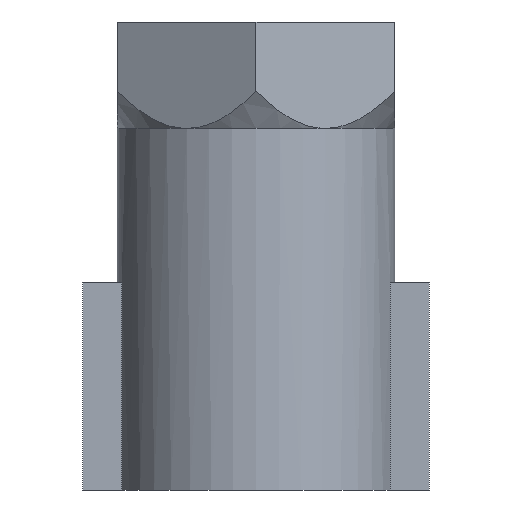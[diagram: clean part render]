
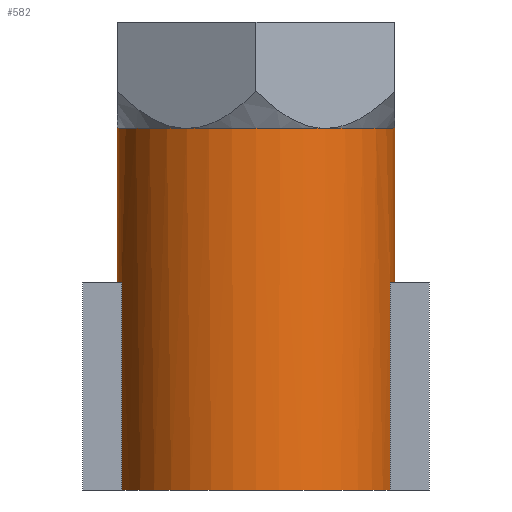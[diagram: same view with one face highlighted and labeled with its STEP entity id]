
A CAD part, front view. The second image highlights one B-rep face of the part: STEP entity #582.
In plain terms, the highlighted cylindrical face has radius 10 mm (diameter 20 mm), a partial arc.
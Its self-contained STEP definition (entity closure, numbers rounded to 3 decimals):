
#63 = VERTEX_POINT ( 'NONE', #501 ) ;
#76 = CARTESIAN_POINT ( 'NONE',  ( 10., 0., 26.075 ) ) ;
#106 = DIRECTION ( 'NONE',  ( 0., 0., -1. ) ) ;
#113 = CARTESIAN_POINT ( 'NONE',  ( 0., 0., 26.075 ) ) ;
#130 = VERTEX_POINT ( 'NONE', #152 ) ;
#152 = CARTESIAN_POINT ( 'NONE',  ( -10., 0., 15. ) ) ;
#212 = DIRECTION ( 'NONE',  ( 1., 0., 0. ) ) ;
#221 = DIRECTION ( 'NONE',  ( 0., 0., 1. ) ) ;
#224 = CARTESIAN_POINT ( 'NONE',  ( 0., 0., 15. ) ) ;
#261 = CIRCLE ( 'NONE', #816, 10. ) ;
#264 = VECTOR ( 'NONE', #981, 1000. ) ;
#270 = DIRECTION ( 'NONE',  ( 0., 0., -1. ) ) ;
#278 = CARTESIAN_POINT ( 'NONE',  ( -10., 0., 16. ) ) ;
#293 = LINE ( 'NONE', #1172, #264 ) ;
#297 = DIRECTION ( 'NONE',  ( 1., 0., 0. ) ) ;
#299 = DIRECTION ( 'NONE',  ( 0., 0., -1. ) ) ;
#300 = CARTESIAN_POINT ( 'NONE',  ( 0., 0., 26.075 ) ) ;
#306 = CARTESIAN_POINT ( 'NONE',  ( 9.682, -2.5, 16. ) ) ;
#316 = DIRECTION ( 'NONE',  ( 0., 0., 1. ) ) ;
#376 = CARTESIAN_POINT ( 'NONE',  ( -10., 0., 26.075 ) ) ;
#411 = DIRECTION ( 'NONE',  ( 1., 0., 0. ) ) ;
#418 = DIRECTION ( 'NONE',  ( 1., 0., 0. ) ) ;
#421 = DIRECTION ( 'NONE',  ( 0., 0., 1. ) ) ;
#422 = EDGE_CURVE ( 'NONE', #63, #885, #925, .T. ) ;
#438 = ORIENTED_EDGE ( 'NONE', *, *, #1187, .F. ) ;
#440 = FACE_OUTER_BOUND ( 'NONE', #640, .T. ) ;
#453 = VECTOR ( 'NONE', #1087, 1000. ) ;
#470 = ORIENTED_EDGE ( 'NONE', *, *, #744, .T. ) ;
#471 = ORIENTED_EDGE ( 'NONE', *, *, #1132, .T. ) ;
#478 = CARTESIAN_POINT ( 'NONE',  ( -9.682, -2.5, 16. ) ) ;
#494 = ORIENTED_EDGE ( 'NONE', *, *, #422, .T. ) ;
#496 = CIRCLE ( 'NONE', #748, 10. ) ;
#501 = CARTESIAN_POINT ( 'NONE',  ( -5., -8.66, 26.075 ) ) ;
#503 = CARTESIAN_POINT ( 'NONE',  ( 0., 0., 0. ) ) ;
#514 = ORIENTED_EDGE ( 'NONE', *, *, #773, .T. ) ;
#516 = ORIENTED_EDGE ( 'NONE', *, *, #1020, .T. ) ;
#582 = ADVANCED_FACE ( 'NONE', ( #440 ), #753, .T. ) ;
#616 = CARTESIAN_POINT ( 'NONE',  ( 9.682, -2.5, 0. ) ) ;
#640 = EDGE_LOOP ( 'NONE', ( #438, #470, #471, #494, #514, #516, #652, #665, #684, #700 ) ) ;
#641 = LINE ( 'NONE', #478, #453 ) ;
#652 = ORIENTED_EDGE ( 'NONE', *, *, #1068, .T. ) ;
#665 = ORIENTED_EDGE ( 'NONE', *, *, #998, .T. ) ;
#684 = ORIENTED_EDGE ( 'NONE', *, *, #933, .T. ) ;
#700 = ORIENTED_EDGE ( 'NONE', *, *, #1140, .T. ) ;
#744 = EDGE_CURVE ( 'NONE', #815, #850, #840, .T. ) ;
#748 = AXIS2_PLACEMENT_3D ( 'NONE', #1095, #1002, #909 ) ;
#753 = CYLINDRICAL_SURFACE ( 'NONE', #889, 10. ) ;
#755 = AXIS2_PLACEMENT_3D ( 'NONE', #113, #106, #411 ) ;
#773 = EDGE_CURVE ( 'NONE', #885, #130, #1169, .T. ) ;
#781 = AXIS2_PLACEMENT_3D ( 'NONE', #224, #221, #212 ) ;
#785 = VECTOR ( 'NONE', #316, 1000. ) ;
#815 = VERTEX_POINT ( 'NONE', #76 ) ;
#816 = AXIS2_PLACEMENT_3D ( 'NONE', #503, #421, #418 ) ;
#820 = CARTESIAN_POINT ( 'NONE',  ( -9.682, -2.5, 0. ) ) ;
#829 = CARTESIAN_POINT ( 'NONE',  ( -9.682, -2.5, 15. ) ) ;
#840 = CIRCLE ( 'NONE', #847, 10. ) ;
#845 = CIRCLE ( 'NONE', #755, 10. ) ;
#846 = DIRECTION ( 'NONE',  ( 0., 0., -1. ) ) ;
#847 = AXIS2_PLACEMENT_3D ( 'NONE', #300, #299, #297 ) ;
#850 = VERTEX_POINT ( 'NONE', #1155 ) ;
#864 = CARTESIAN_POINT ( 'NONE',  ( 10., 0., 15. ) ) ;
#878 = VERTEX_POINT ( 'NONE', #864 ) ;
#885 = VERTEX_POINT ( 'NONE', #376 ) ;
#889 = AXIS2_PLACEMENT_3D ( 'NONE', #894, #846, #897 ) ;
#894 = CARTESIAN_POINT ( 'NONE',  ( 0., 0., 16. ) ) ;
#897 = DIRECTION ( 'NONE',  ( -1., 0., 0. ) ) ;
#909 = DIRECTION ( 'NONE',  ( 1., 0., 0. ) ) ;
#925 = CIRCLE ( 'NONE', #1103, 10. ) ;
#933 = EDGE_CURVE ( 'NONE', #1123, #1075, #957, .T. ) ;
#935 = CARTESIAN_POINT ( 'NONE',  ( 0., 0., 26.075 ) ) ;
#942 = DIRECTION ( 'NONE',  ( 0., 0., -1. ) ) ;
#944 = DIRECTION ( 'NONE',  ( 1., 0., 0. ) ) ;
#952 = VECTOR ( 'NONE', #270, 1000. ) ;
#957 = LINE ( 'NONE', #306, #785 ) ;
#981 = DIRECTION ( 'NONE',  ( 0., 0., -1. ) ) ;
#991 = VERTEX_POINT ( 'NONE', #829 ) ;
#998 = EDGE_CURVE ( 'NONE', #1111, #1123, #261, .T. ) ;
#1002 = DIRECTION ( 'NONE',  ( 0., 0., 1. ) ) ;
#1020 = EDGE_CURVE ( 'NONE', #130, #991, #1127, .T. ) ;
#1068 = EDGE_CURVE ( 'NONE', #991, #1111, #641, .T. ) ;
#1075 = VERTEX_POINT ( 'NONE', #1189 ) ;
#1087 = DIRECTION ( 'NONE',  ( 0., 0., -1. ) ) ;
#1095 = CARTESIAN_POINT ( 'NONE',  ( 0., 0., 15. ) ) ;
#1103 = AXIS2_PLACEMENT_3D ( 'NONE', #935, #942, #944 ) ;
#1111 = VERTEX_POINT ( 'NONE', #820 ) ;
#1123 = VERTEX_POINT ( 'NONE', #616 ) ;
#1127 = CIRCLE ( 'NONE', #781, 10. ) ;
#1132 = EDGE_CURVE ( 'NONE', #850, #63, #845, .T. ) ;
#1140 = EDGE_CURVE ( 'NONE', #1075, #878, #496, .T. ) ;
#1155 = CARTESIAN_POINT ( 'NONE',  ( 5., -8.66, 26.075 ) ) ;
#1169 = LINE ( 'NONE', #278, #952 ) ;
#1172 = CARTESIAN_POINT ( 'NONE',  ( 10., 0., 16. ) ) ;
#1187 = EDGE_CURVE ( 'NONE', #815, #878, #293, .T. ) ;
#1189 = CARTESIAN_POINT ( 'NONE',  ( 9.682, -2.5, 15. ) ) ;
